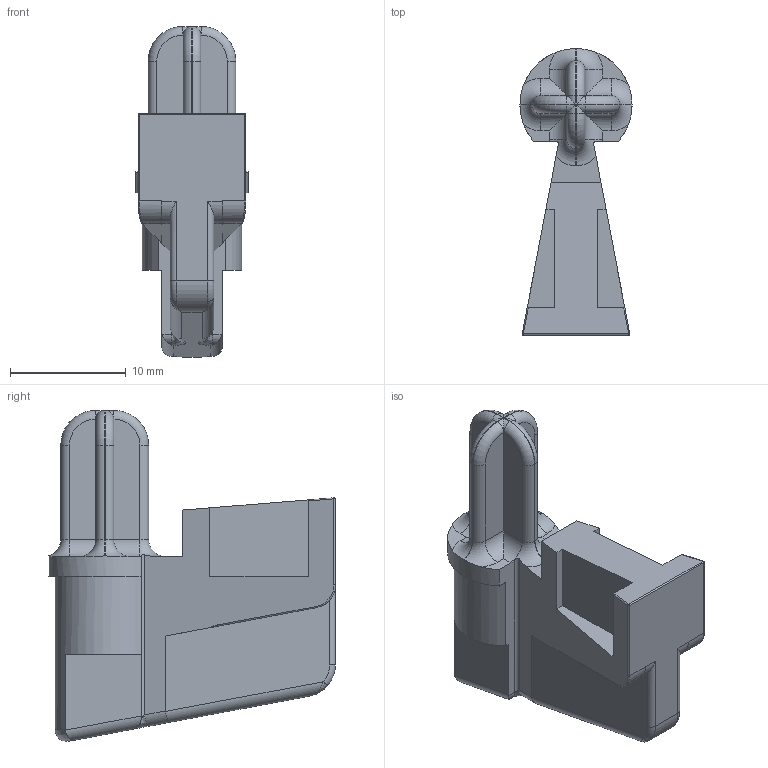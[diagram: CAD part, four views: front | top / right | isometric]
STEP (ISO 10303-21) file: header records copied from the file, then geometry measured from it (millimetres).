
FILE_DESCRIPTION(/* description */ (''),/* implementation_level */ '2;1');
FILE_NAME(/* name */ 'Follower-v3.step.step',/* time_stamp */ '2021-06-23T20:44:01-07:00',/* author */ (''),/* organization */ (''),/* preprocessor_version */ 'ST-DEVELOPER v18.1',/* originating_system */ 'Autodesk Translation Framework v10.9.0.1377',/* authorisation */ '');
FILE_SCHEMA (('AUTOMOTIVE_DESIGN { 1 0 10303 214 3 1 1 }'));
Length unit declared in the file: millimetre
Products named in the file (1): cmmg-25 round-Follower v6
Bounding box: 9.7 x 24.8 x 28.63 mm (x, y, z)
Volume: 2251.4 mm3; surface area: 1698.4 mm2
Topology: 1 solids, 1 shells, 140 faces, 361 edges, 216 vertices
Faces by surface type: cylinder 60, plane 50, torus 18, bspline 10, sphere 2
Entity records: 4660 total; most frequent: CARTESIAN_POINT 1273, DIRECTION 724, ORIENTED_EDGE 700, EDGE_CURVE 350, AXIS2_PLACEMENT_3D 273, VERTEX_POINT 212, LINE 178, VECTOR 178
